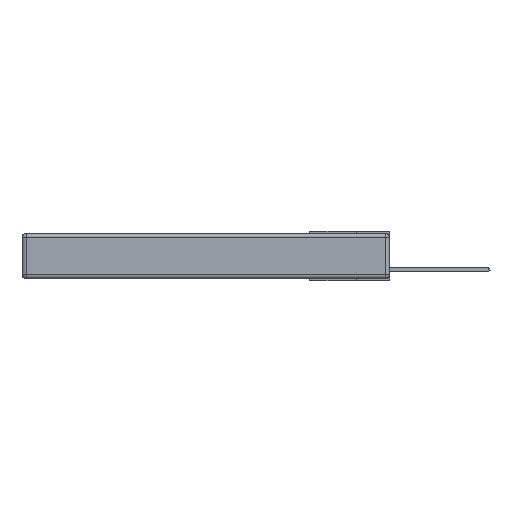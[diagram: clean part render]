
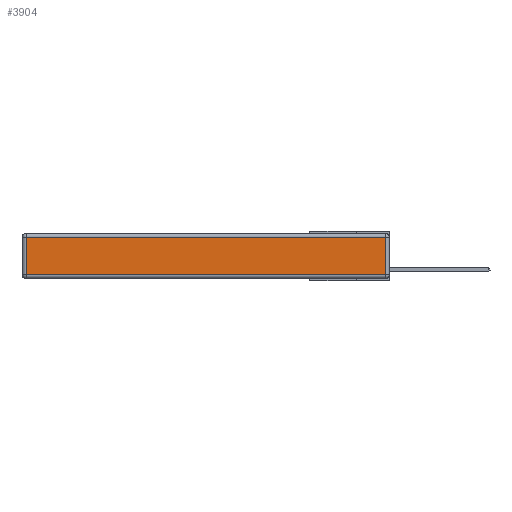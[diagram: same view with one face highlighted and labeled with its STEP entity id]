
A CAD part, left-side view. The second image highlights one B-rep face of the part: STEP entity #3904.
In plain terms, the highlighted planar face has unit normal (-1, 0, 0).
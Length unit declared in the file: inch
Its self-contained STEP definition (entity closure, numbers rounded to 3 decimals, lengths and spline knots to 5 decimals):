
#3734 = VERTEX_POINT ( 'NONE', #9882 ) ;
#3784 = DIRECTION ( 'NONE',  ( -1., 0., 0. ) ) ;
#3904 = ADVANCED_FACE ( 'NONE', ( #30071 ), #26632, .T. ) ;
#5282 = EDGE_CURVE ( 'NONE', #24483, #3734, #22778, .T. ) ;
#5844 = VERTEX_POINT ( 'NONE', #23517 ) ;
#6268 = CARTESIAN_POINT ( 'NONE',  ( 0., 0., -0.343 ) ) ;
#7135 = DIRECTION ( 'NONE',  ( 0., 0., -1. ) ) ;
#8300 = ORIENTED_EDGE ( 'NONE', *, *, #5282, .T. ) ;
#9882 = CARTESIAN_POINT ( 'NONE',  ( 0., 0.03, -0.03 ) ) ;
#9986 = VECTOR ( 'NONE', #22771, 39.37008 ) ;
#10869 = VECTOR ( 'NONE', #7135, 39.37008 ) ;
#11128 = EDGE_CURVE ( 'NONE', #3734, #5844, #14232, .T. ) ;
#13307 = DIRECTION ( 'NONE',  ( 0., 1., 0. ) ) ;
#13412 = CARTESIAN_POINT ( 'NONE',  ( 0., 2.75, -0.03 ) ) ;
#13713 = ORIENTED_EDGE ( 'NONE', *, *, #11128, .T. ) ;
#13786 = DIRECTION ( 'NONE',  ( 0., 0., 1. ) ) ;
#14232 = LINE ( 'NONE', #13412, #23041 ) ;
#14544 = CARTESIAN_POINT ( 'NONE',  ( 0., 2.72, -0.313 ) ) ;
#15178 = CARTESIAN_POINT ( 'NONE',  ( 0., 0.03, -0.343 ) ) ;
#15263 = LINE ( 'NONE', #32758, #10869 ) ;
#18603 = CARTESIAN_POINT ( 'NONE',  ( 0., 0.03, -0.313 ) ) ;
#19801 = ORIENTED_EDGE ( 'NONE', *, *, #27364, .T. ) ;
#21116 = DIRECTION ( 'NONE',  ( 0., 0., 1. ) ) ;
#21973 = AXIS2_PLACEMENT_3D ( 'NONE', #6268, #3784, #13786 ) ;
#22771 = DIRECTION ( 'NONE',  ( 0., -1., 0. ) ) ;
#22778 = LINE ( 'NONE', #15178, #30342 ) ;
#23041 = VECTOR ( 'NONE', #13307, 39.37008 ) ;
#23517 = CARTESIAN_POINT ( 'NONE',  ( 0., 2.72, -0.03 ) ) ;
#23627 = LINE ( 'NONE', #25361, #9986 ) ;
#24483 = VERTEX_POINT ( 'NONE', #18603 ) ;
#25361 = CARTESIAN_POINT ( 'NONE',  ( 0., 0., -0.313 ) ) ;
#25633 = EDGE_LOOP ( 'NONE', ( #19801, #8300, #13713, #26386 ) ) ;
#26386 = ORIENTED_EDGE ( 'NONE', *, *, #32171, .T. ) ;
#26632 = PLANE ( 'NONE',  #21973 ) ;
#27364 = EDGE_CURVE ( 'NONE', #28094, #24483, #23627, .T. ) ;
#28094 = VERTEX_POINT ( 'NONE', #14544 ) ;
#30071 = FACE_OUTER_BOUND ( 'NONE', #25633, .T. ) ;
#30342 = VECTOR ( 'NONE', #21116, 39.37008 ) ;
#32171 = EDGE_CURVE ( 'NONE', #5844, #28094, #15263, .T. ) ;
#32758 = CARTESIAN_POINT ( 'NONE',  ( 0., 2.72, -0.343 ) ) ;
